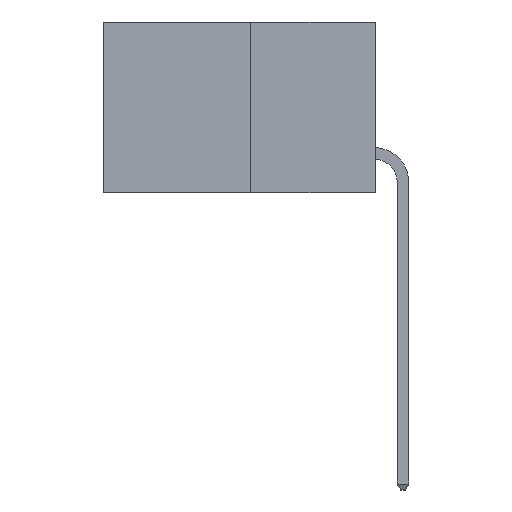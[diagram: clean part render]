
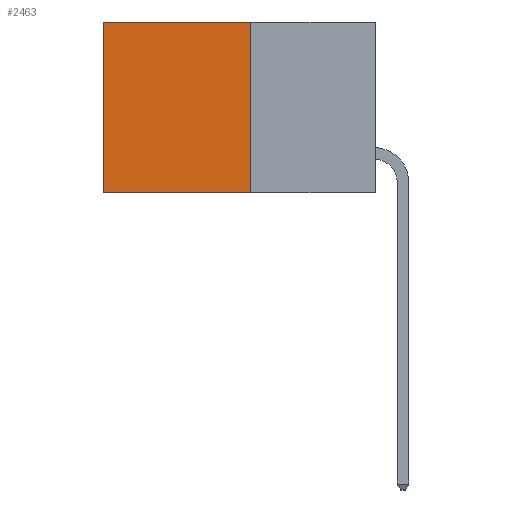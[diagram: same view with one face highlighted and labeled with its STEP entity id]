
A CAD part, left-side view. The second image highlights one B-rep face of the part: STEP entity #2463.
In plain terms, the highlighted planar face has unit normal (-1, 0, 0).
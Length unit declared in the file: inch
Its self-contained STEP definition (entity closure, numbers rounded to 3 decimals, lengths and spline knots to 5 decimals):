
#12 = DIRECTION ( 'NONE',  ( 0., 1., 0. ) ) ;
#1049 = CARTESIAN_POINT ( 'NONE',  ( 0.277, 0.59, -0.37 ) ) ;
#1157 = DIRECTION ( 'NONE',  ( 0., 0., -1. ) ) ;
#1573 = ORIENTED_EDGE ( 'NONE', *, *, #3918, .T. ) ;
#1622 = PLANE ( 'NONE',  #12481 ) ;
#1774 = CARTESIAN_POINT ( 'NONE',  ( 0.277, 0.27, -0.37 ) ) ;
#1818 = CARTESIAN_POINT ( 'NONE',  ( 0.277, 0.27, 0. ) ) ;
#2129 = VERTEX_POINT ( 'NONE', #1818 ) ;
#2463 = ADVANCED_FACE ( 'NONE', ( #9412 ), #1622, .F. ) ;
#2584 = LINE ( 'NONE', #1049, #7720 ) ;
#2940 = VERTEX_POINT ( 'NONE', #7010 ) ;
#3635 = DIRECTION ( 'NONE',  ( 0., 0., -1. ) ) ;
#3918 = EDGE_CURVE ( 'NONE', #2940, #6933, #2584, .T. ) ;
#4842 = DIRECTION ( 'NONE',  ( 0., 1., 0. ) ) ;
#5603 = VECTOR ( 'NONE', #12, 39.37008 ) ;
#6118 = EDGE_CURVE ( 'NONE', #2129, #2940, #11091, .T. ) ;
#6850 = DIRECTION ( 'NONE',  ( 0., 0., -1. ) ) ;
#6877 = DIRECTION ( 'NONE',  ( 1., 0., 0. ) ) ;
#6933 = VERTEX_POINT ( 'NONE', #12255 ) ;
#7010 = CARTESIAN_POINT ( 'NONE',  ( 0.277, 0.59, 0. ) ) ;
#7190 = CARTESIAN_POINT ( 'NONE',  ( 0.277, 0.27, 0. ) ) ;
#7480 = LINE ( 'NONE', #11973, #12834 ) ;
#7683 = CARTESIAN_POINT ( 'NONE',  ( 0.277, 0.27, -0.37 ) ) ;
#7720 = VECTOR ( 'NONE', #1157, 39.37008 ) ;
#9234 = VECTOR ( 'NONE', #3635, 39.37008 ) ;
#9412 = FACE_OUTER_BOUND ( 'NONE', #9960, .T. ) ;
#9503 = VERTEX_POINT ( 'NONE', #1774 ) ;
#9555 = ORIENTED_EDGE ( 'NONE', *, *, #6118, .T. ) ;
#9960 = EDGE_LOOP ( 'NONE', ( #1573, #12472, #11428, #9555 ) ) ;
#10836 = EDGE_CURVE ( 'NONE', #2129, #9503, #11870, .T. ) ;
#10841 = CARTESIAN_POINT ( 'NONE',  ( 0.277, 0.27, -0.37 ) ) ;
#11091 = LINE ( 'NONE', #7190, #5603 ) ;
#11428 = ORIENTED_EDGE ( 'NONE', *, *, #10836, .F. ) ;
#11870 = LINE ( 'NONE', #10841, #9234 ) ;
#11973 = CARTESIAN_POINT ( 'NONE',  ( 0.277, 0.27, -0.37 ) ) ;
#12255 = CARTESIAN_POINT ( 'NONE',  ( 0.277, 0.59, -0.37 ) ) ;
#12472 = ORIENTED_EDGE ( 'NONE', *, *, #12765, .F. ) ;
#12481 = AXIS2_PLACEMENT_3D ( 'NONE', #7683, #6877, #6850 ) ;
#12765 = EDGE_CURVE ( 'NONE', #9503, #6933, #7480, .T. ) ;
#12834 = VECTOR ( 'NONE', #4842, 39.37008 ) ;
